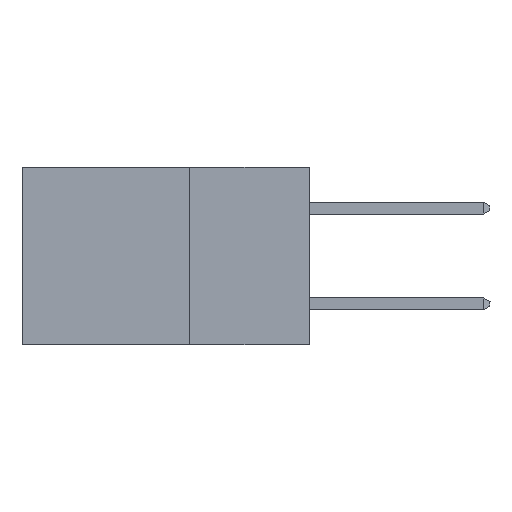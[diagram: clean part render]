
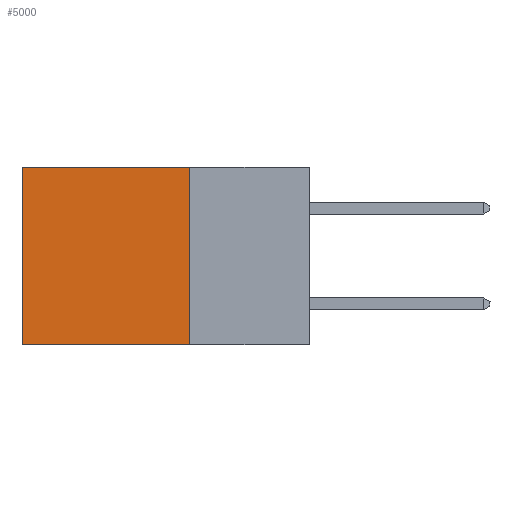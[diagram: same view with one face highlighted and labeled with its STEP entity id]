
A CAD part, left-side view. The second image highlights one B-rep face of the part: STEP entity #5000.
In plain terms, the highlighted planar face has unit normal (-1, 0, 0).
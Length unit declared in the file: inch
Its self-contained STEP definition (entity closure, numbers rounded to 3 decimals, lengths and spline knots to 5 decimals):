
#161 = EDGE_CURVE ( 'NONE', #9145, #25242, #28986, .T. ) ;
#2771 = DIRECTION ( 'NONE',  ( 0., 1., 0. ) ) ;
#2854 = DIRECTION ( 'NONE',  ( 1., 0., 0. ) ) ;
#3077 = PLANE ( 'NONE',  #29664 ) ;
#3178 = DIRECTION ( 'NONE',  ( 0., 1., 0. ) ) ;
#5000 = ADVANCED_FACE ( 'NONE', ( #24002 ), #3077, .F. ) ;
#5730 = CARTESIAN_POINT ( 'NONE',  ( 0.2875, 0.25, 0. ) ) ;
#8002 = ORIENTED_EDGE ( 'NONE', *, *, #161, .T. ) ;
#9065 = VECTOR ( 'NONE', #2771, 39.37008 ) ;
#9145 = VERTEX_POINT ( 'NONE', #9721 ) ;
#9372 = VERTEX_POINT ( 'NONE', #24412 ) ;
#9721 = CARTESIAN_POINT ( 'NONE',  ( 0.2875, 0.25, 0. ) ) ;
#12331 = LINE ( 'NONE', #28083, #34075 ) ;
#12363 = CARTESIAN_POINT ( 'NONE',  ( 0.2875, 0.6, -0.37 ) ) ;
#17221 = DIRECTION ( 'NONE',  ( 0., 0., -1. ) ) ;
#19209 = LINE ( 'NONE', #27517, #35502 ) ;
#19903 = CARTESIAN_POINT ( 'NONE',  ( 0.2875, 0.25, -0.37 ) ) ;
#20920 = ORIENTED_EDGE ( 'NONE', *, *, #33224, .T. ) ;
#20953 = ORIENTED_EDGE ( 'NONE', *, *, #35357, .F. ) ;
#24002 = FACE_OUTER_BOUND ( 'NONE', #29821, .T. ) ;
#24412 = CARTESIAN_POINT ( 'NONE',  ( 0.2875, 0.25, -0.37 ) ) ;
#24926 = LINE ( 'NONE', #19903, #9065 ) ;
#25242 = VERTEX_POINT ( 'NONE', #36838 ) ;
#25741 = ORIENTED_EDGE ( 'NONE', *, *, #36237, .F. ) ;
#27517 = CARTESIAN_POINT ( 'NONE',  ( 0.2875, 0.6, 0. ) ) ;
#27700 = DIRECTION ( 'NONE',  ( 0., 0., -1. ) ) ;
#28083 = CARTESIAN_POINT ( 'NONE',  ( 0.2875, 0.25, 0. ) ) ;
#28986 = LINE ( 'NONE', #32236, #34406 ) ;
#29664 = AXIS2_PLACEMENT_3D ( 'NONE', #5730, #2854, #17221 ) ;
#29821 = EDGE_LOOP ( 'NONE', ( #20920, #25741, #20953, #8002 ) ) ;
#30558 = DIRECTION ( 'NONE',  ( 0., 0., -1. ) ) ;
#32236 = CARTESIAN_POINT ( 'NONE',  ( 0.2875, 0.25, 0. ) ) ;
#33224 = EDGE_CURVE ( 'NONE', #25242, #35827, #19209, .T. ) ;
#34075 = VECTOR ( 'NONE', #27700, 39.37008 ) ;
#34406 = VECTOR ( 'NONE', #3178, 39.37008 ) ;
#35357 = EDGE_CURVE ( 'NONE', #9145, #9372, #12331, .T. ) ;
#35502 = VECTOR ( 'NONE', #30558, 39.37008 ) ;
#35827 = VERTEX_POINT ( 'NONE', #12363 ) ;
#36237 = EDGE_CURVE ( 'NONE', #9372, #35827, #24926, .T. ) ;
#36838 = CARTESIAN_POINT ( 'NONE',  ( 0.2875, 0.6, 0. ) ) ;
